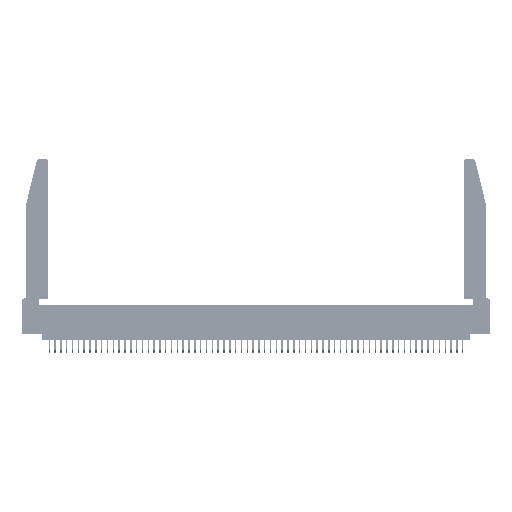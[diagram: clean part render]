
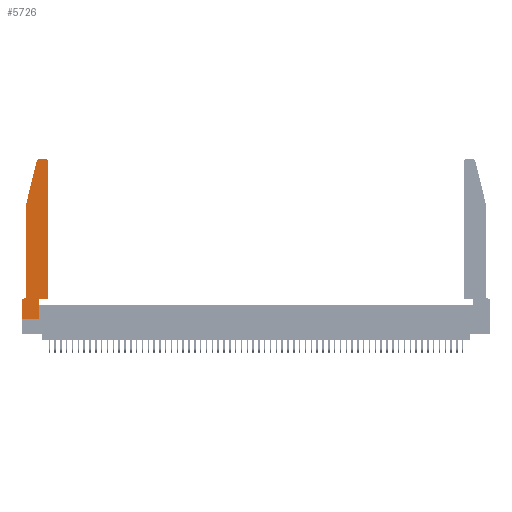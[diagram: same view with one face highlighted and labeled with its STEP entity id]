
A CAD part, top view. The second image highlights one B-rep face of the part: STEP entity #5726.
In plain terms, the highlighted planar face has unit normal (0, 0, 1).
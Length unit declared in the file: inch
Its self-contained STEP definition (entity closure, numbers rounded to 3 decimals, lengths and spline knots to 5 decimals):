
#210 = EDGE_CURVE ( 'NONE', #7356, #13680, #16972, .T. ) ;
#1644 = AXIS2_PLACEMENT_3D ( 'NONE', #47877, #16006, #2429 ) ;
#2429 = DIRECTION ( 'NONE',  ( 1., 0., 0. ) ) ;
#2516 = ORIENTED_EDGE ( 'NONE', *, *, #3280, .T. ) ;
#3280 = EDGE_CURVE ( 'NONE', #27470, #14948, #51471, .T. ) ;
#4256 = VERTEX_POINT ( 'NONE', #15973 ) ;
#4704 = CARTESIAN_POINT ( 'NONE',  ( 0.25487, 2.72718, 0.37 ) ) ;
#5359 = FACE_OUTER_BOUND ( 'NONE', #17509, .T. ) ;
#5726 = ADVANCED_FACE ( 'NONE', ( #5359 ), #23507, .T. ) ;
#5929 = CARTESIAN_POINT ( 'NONE',  ( 0.0755, 2., 0.37 ) ) ;
#6092 = CARTESIAN_POINT ( 'NONE',  ( 0.4505, 0.35, 0.37 ) ) ;
#7356 = VERTEX_POINT ( 'NONE', #53312 ) ;
#7489 = ORIENTED_EDGE ( 'NONE', *, *, #34560, .T. ) ;
#9001 = EDGE_CURVE ( 'NONE', #9279, #28495, #44306, .T. ) ;
#9050 = ORIENTED_EDGE ( 'NONE', *, *, #57700, .T. ) ;
#9279 = VERTEX_POINT ( 'NONE', #22924 ) ;
#9856 = ORIENTED_EDGE ( 'NONE', *, *, #23206, .T. ) ;
#10335 = VECTOR ( 'NONE', #52804, 39.37008 ) ;
#11043 = LINE ( 'NONE', #50169, #52331 ) ;
#13037 = DIRECTION ( 'NONE',  ( -1., 0., 0. ) ) ;
#13282 = CARTESIAN_POINT ( 'NONE',  ( 0.4505, 0.35, 0.37 ) ) ;
#13680 = VERTEX_POINT ( 'NONE', #58634 ) ;
#14645 = EDGE_CURVE ( 'NONE', #28495, #23687, #40026, .T. ) ;
#14948 = VERTEX_POINT ( 'NONE', #21479 ) ;
#15853 = DIRECTION ( 'NONE',  ( 0., 1., 0. ) ) ;
#15973 = CARTESIAN_POINT ( 'NONE',  ( 0.0755, 0.42, 0.37 ) ) ;
#16006 = DIRECTION ( 'NONE',  ( 0., 0., 1. ) ) ;
#16972 = LINE ( 'NONE', #56993, #21228 ) ;
#17509 = EDGE_LOOP ( 'NONE', ( #22402, #9050, #9856, #57268, #21498, #17693, #2516, #7489, #17855, #48972, #39360, #20340 ) ) ;
#17558 = VECTOR ( 'NONE', #39904, 39.37008 ) ;
#17586 = CIRCLE ( 'NONE', #23967, 0.07 ) ;
#17693 = ORIENTED_EDGE ( 'NONE', *, *, #33029, .T. ) ;
#17855 = ORIENTED_EDGE ( 'NONE', *, *, #210, .T. ) ;
#17998 = DIRECTION ( 'NONE',  ( 1., 0., 0. ) ) ;
#18146 = CARTESIAN_POINT ( 'NONE',  ( 0.0755, 2., 0.37 ) ) ;
#20340 = ORIENTED_EDGE ( 'NONE', *, *, #9001, .T. ) ;
#21228 = VECTOR ( 'NONE', #50056, 39.37008 ) ;
#21479 = CARTESIAN_POINT ( 'NONE',  ( 0., 0., 0.37 ) ) ;
#21498 = ORIENTED_EDGE ( 'NONE', *, *, #42395, .T. ) ;
#22402 = ORIENTED_EDGE ( 'NONE', *, *, #14645, .T. ) ;
#22426 = LINE ( 'NONE', #30882, #10335 ) ;
#22924 = CARTESIAN_POINT ( 'NONE',  ( 0.4505, 2.72, 0.37 ) ) ;
#22933 = DIRECTION ( 'NONE',  ( 0., 0., 1. ) ) ;
#23206 = EDGE_CURVE ( 'NONE', #53605, #40402, #56835, .T. ) ;
#23507 = PLANE ( 'NONE',  #29398 ) ;
#23687 = VERTEX_POINT ( 'NONE', #36681 ) ;
#23967 = AXIS2_PLACEMENT_3D ( 'NONE', #25775, #35098, #13037 ) ;
#24279 = DIRECTION ( 'NONE',  ( -1., 0., 0. ) ) ;
#25179 = VERTEX_POINT ( 'NONE', #38763 ) ;
#25775 = CARTESIAN_POINT ( 'NONE',  ( 0.0055, 0.42, 0.37 ) ) ;
#26808 = DIRECTION ( 'NONE',  ( 0., -1., 0. ) ) ;
#27470 = VERTEX_POINT ( 'NONE', #54236 ) ;
#28495 = VERTEX_POINT ( 'NONE', #48177 ) ;
#29027 = AXIS2_PLACEMENT_3D ( 'NONE', #36237, #41472, #17998 ) ;
#29398 = AXIS2_PLACEMENT_3D ( 'NONE', #36624, #22933, #55362 ) ;
#30763 = VECTOR ( 'NONE', #24279, 39.37008 ) ;
#30882 = CARTESIAN_POINT ( 'NONE',  ( 0., 0., 0.37 ) ) ;
#31528 = CARTESIAN_POINT ( 'NONE',  ( 0.4505, 0.35, 0.37 ) ) ;
#32109 = LINE ( 'NONE', #6092, #41385 ) ;
#33029 = EDGE_CURVE ( 'NONE', #25179, #27470, #33986, .T. ) ;
#33557 = DIRECTION ( 'NONE',  ( -0.239, -0.971, 0. ) ) ;
#33986 = LINE ( 'NONE', #38424, #51855 ) ;
#34560 = EDGE_CURVE ( 'NONE', #14948, #7356, #22426, .T. ) ;
#35098 = DIRECTION ( 'NONE',  ( 0., 0., -1. ) ) ;
#36237 = CARTESIAN_POINT ( 'NONE',  ( 0.284, 2.72, 0.37 ) ) ;
#36624 = CARTESIAN_POINT ( 'NONE',  ( 0., 0.35, 0.37 ) ) ;
#36681 = CARTESIAN_POINT ( 'NONE',  ( 0.284, 2.75, 0.37 ) ) ;
#38424 = CARTESIAN_POINT ( 'NONE',  ( 0.0755, 0.35, 0.37 ) ) ;
#38763 = CARTESIAN_POINT ( 'NONE',  ( 0.0055, 0.35, 0.37 ) ) ;
#39360 = ORIENTED_EDGE ( 'NONE', *, *, #51372, .T. ) ;
#39904 = DIRECTION ( 'NONE',  ( 1., 0., 0. ) ) ;
#40026 = LINE ( 'NONE', #51581, #30763 ) ;
#40402 = VERTEX_POINT ( 'NONE', #18146 ) ;
#41385 = VECTOR ( 'NONE', #15853, 39.37008 ) ;
#41472 = DIRECTION ( 'NONE',  ( 0., 0., 1. ) ) ;
#42395 = EDGE_CURVE ( 'NONE', #4256, #25179, #17586, .T. ) ;
#42418 = EDGE_CURVE ( 'NONE', #13680, #51294, #55303, .T. ) ;
#42710 = CIRCLE ( 'NONE', #29027, 0.03 ) ;
#44306 = CIRCLE ( 'NONE', #1644, 0.03 ) ;
#47877 = CARTESIAN_POINT ( 'NONE',  ( 0.4205, 2.72, 0.37 ) ) ;
#48177 = CARTESIAN_POINT ( 'NONE',  ( 0.4205, 2.75, 0.37 ) ) ;
#48644 = VECTOR ( 'NONE', #26808, 39.37008 ) ;
#48972 = ORIENTED_EDGE ( 'NONE', *, *, #42418, .T. ) ;
#49366 = EDGE_CURVE ( 'NONE', #40402, #4256, #11043, .T. ) ;
#50056 = DIRECTION ( 'NONE',  ( 0., 1., 0. ) ) ;
#50169 = CARTESIAN_POINT ( 'NONE',  ( 0.0755, 2., 0.37 ) ) ;
#51294 = VERTEX_POINT ( 'NONE', #13282 ) ;
#51372 = EDGE_CURVE ( 'NONE', #51294, #9279, #32109, .T. ) ;
#51471 = LINE ( 'NONE', #54082, #48644 ) ;
#51581 = CARTESIAN_POINT ( 'NONE',  ( 0.2605, 2.75, 0.37 ) ) ;
#51855 = VECTOR ( 'NONE', #52177, 39.37008 ) ;
#52177 = DIRECTION ( 'NONE',  ( -1., 0., 0. ) ) ;
#52331 = VECTOR ( 'NONE', #54331, 39.37008 ) ;
#52804 = DIRECTION ( 'NONE',  ( 1., 0., 0. ) ) ;
#53312 = CARTESIAN_POINT ( 'NONE',  ( 0.2865, 0., 0.37 ) ) ;
#53605 = VERTEX_POINT ( 'NONE', #4704 ) ;
#54082 = CARTESIAN_POINT ( 'NONE',  ( 0., 0., 0.37 ) ) ;
#54236 = CARTESIAN_POINT ( 'NONE',  ( 0., 0.35, 0.37 ) ) ;
#54331 = DIRECTION ( 'NONE',  ( 0., -1., 0. ) ) ;
#55303 = LINE ( 'NONE', #31528, #17558 ) ;
#55362 = DIRECTION ( 'NONE',  ( 1., 0., 0. ) ) ;
#56835 = LINE ( 'NONE', #5929, #58200 ) ;
#56993 = CARTESIAN_POINT ( 'NONE',  ( 0.2865, 0.35, 0.37 ) ) ;
#57268 = ORIENTED_EDGE ( 'NONE', *, *, #49366, .T. ) ;
#57700 = EDGE_CURVE ( 'NONE', #23687, #53605, #42710, .T. ) ;
#58200 = VECTOR ( 'NONE', #33557, 39.37008 ) ;
#58634 = CARTESIAN_POINT ( 'NONE',  ( 0.2865, 0.35, 0.37 ) ) ;
